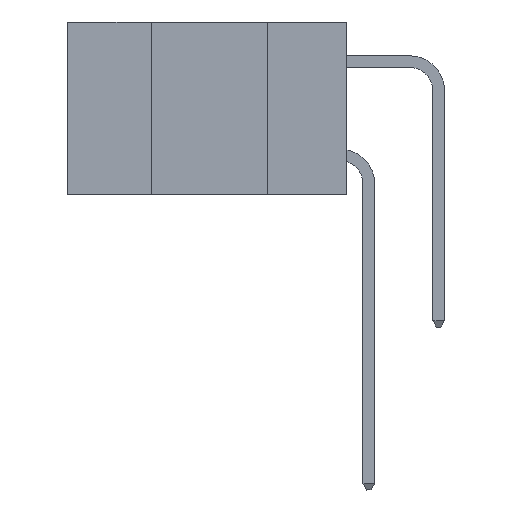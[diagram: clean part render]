
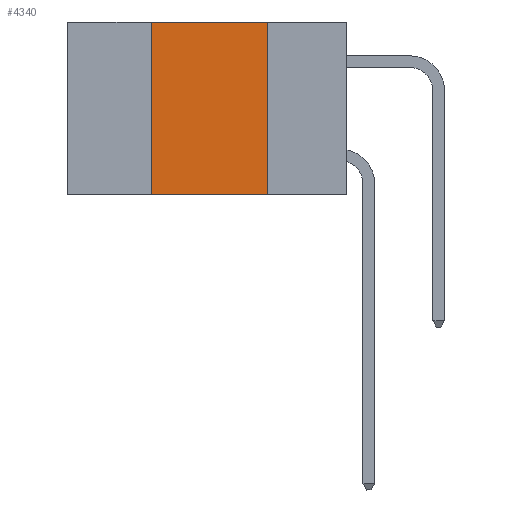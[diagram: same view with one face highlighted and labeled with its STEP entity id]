
A CAD part, left-side view. The second image highlights one B-rep face of the part: STEP entity #4340.
In plain terms, the highlighted planar face has unit normal (-1, 0, 0).
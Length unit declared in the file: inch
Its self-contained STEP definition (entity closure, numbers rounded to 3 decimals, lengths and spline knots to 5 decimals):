
#121 = EDGE_CURVE ( 'NONE', #21773, #1303, #14176, .T. ) ;
#290 = LINE ( 'NONE', #5869, #6733 ) ;
#1297 = ORIENTED_EDGE ( 'NONE', *, *, #4784, .F. ) ;
#1303 = VERTEX_POINT ( 'NONE', #19472 ) ;
#2300 = VECTOR ( 'NONE', #25956, 39.37008 ) ;
#2500 = CARTESIAN_POINT ( 'NONE',  ( 0., 0.42, -0.37 ) ) ;
#3914 = AXIS2_PLACEMENT_3D ( 'NONE', #8545, #17286, #21380 ) ;
#4340 = ADVANCED_FACE ( 'NONE', ( #22687 ), #27827, .F. ) ;
#4784 = EDGE_CURVE ( 'NONE', #7203, #1303, #290, .T. ) ;
#5869 = CARTESIAN_POINT ( 'NONE',  ( 0., 0.17, 0. ) ) ;
#6203 = VERTEX_POINT ( 'NONE', #22185 ) ;
#6733 = VECTOR ( 'NONE', #22888, 39.37008 ) ;
#7203 = VERTEX_POINT ( 'NONE', #15856 ) ;
#7797 = VECTOR ( 'NONE', #28046, 39.37008 ) ;
#8124 = LINE ( 'NONE', #8518, #2300 ) ;
#8402 = ORIENTED_EDGE ( 'NONE', *, *, #9152, .F. ) ;
#8518 = CARTESIAN_POINT ( 'NONE',  ( 0., 0.6, 0. ) ) ;
#8545 = CARTESIAN_POINT ( 'NONE',  ( 0., 0.6, 0. ) ) ;
#9152 = EDGE_CURVE ( 'NONE', #21773, #6203, #21694, .T. ) ;
#10435 = VECTOR ( 'NONE', #27400, 39.37008 ) ;
#14176 = LINE ( 'NONE', #19458, #10435 ) ;
#15856 = CARTESIAN_POINT ( 'NONE',  ( 0., 0.17, 0. ) ) ;
#16047 = ORIENTED_EDGE ( 'NONE', *, *, #19369, .F. ) ;
#17286 = DIRECTION ( 'NONE',  ( 1., 0., 0. ) ) ;
#18441 = CARTESIAN_POINT ( 'NONE',  ( 0., 0.42, 0. ) ) ;
#19369 = EDGE_CURVE ( 'NONE', #6203, #7203, #8124, .T. ) ;
#19458 = CARTESIAN_POINT ( 'NONE',  ( 0., 0.6, -0.37 ) ) ;
#19472 = CARTESIAN_POINT ( 'NONE',  ( 0., 0.17, -0.37 ) ) ;
#21380 = DIRECTION ( 'NONE',  ( 0., 0., -1. ) ) ;
#21694 = LINE ( 'NONE', #18441, #7797 ) ;
#21710 = ORIENTED_EDGE ( 'NONE', *, *, #121, .T. ) ;
#21773 = VERTEX_POINT ( 'NONE', #2500 ) ;
#22185 = CARTESIAN_POINT ( 'NONE',  ( 0., 0.42, 0. ) ) ;
#22687 = FACE_OUTER_BOUND ( 'NONE', #23808, .T. ) ;
#22888 = DIRECTION ( 'NONE',  ( 0., 0., -1. ) ) ;
#23808 = EDGE_LOOP ( 'NONE', ( #1297, #16047, #8402, #21710 ) ) ;
#25956 = DIRECTION ( 'NONE',  ( 0., -1., 0. ) ) ;
#27400 = DIRECTION ( 'NONE',  ( 0., -1., 0. ) ) ;
#27827 = PLANE ( 'NONE',  #3914 ) ;
#28046 = DIRECTION ( 'NONE',  ( 0., 0., 1. ) ) ;
